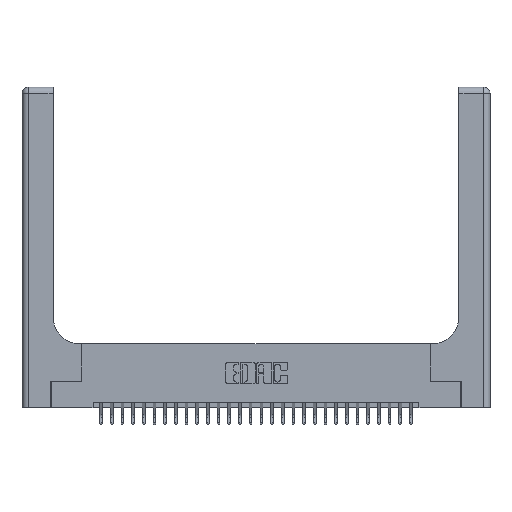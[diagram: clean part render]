
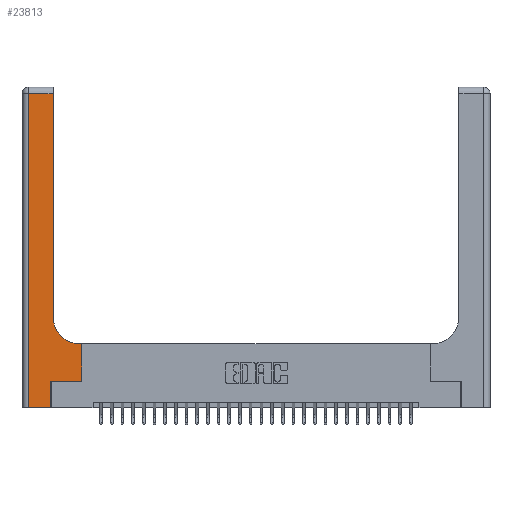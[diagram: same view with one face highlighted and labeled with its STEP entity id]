
A CAD part, top view. The second image highlights one B-rep face of the part: STEP entity #23813.
In plain terms, the highlighted planar face has unit normal (0, 0, 1).
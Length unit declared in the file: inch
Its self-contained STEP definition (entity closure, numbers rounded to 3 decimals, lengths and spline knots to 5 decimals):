
#58 = VERTEX_POINT ( 'NONE', #15473 ) ;
#102 = DIRECTION ( 'NONE',  ( 0., 1., 0. ) ) ;
#918 = AXIS2_PLACEMENT_3D ( 'NONE', #6945, #30186, #16162 ) ;
#1319 = CARTESIAN_POINT ( 'NONE',  ( 0.5415, 0.6, 0.37 ) ) ;
#1729 = CARTESIAN_POINT ( 'NONE',  ( 0.06, 3., 0.37 ) ) ;
#1959 = LINE ( 'NONE', #2387, #11537 ) ;
#2387 = CARTESIAN_POINT ( 'NONE',  ( 0.5585, 0.25, 0.37 ) ) ;
#2686 = VERTEX_POINT ( 'NONE', #16054 ) ;
#3421 = EDGE_LOOP ( 'NONE', ( #17281, #29422, #12052, #12313, #5362, #10881, #8377, #27648, #24285 ) ) ;
#3816 = CARTESIAN_POINT ( 'NONE',  ( 0.269, 0., 0.37 ) ) ;
#3995 = CIRCLE ( 'NONE', #918, 0.25 ) ;
#4967 = EDGE_CURVE ( 'NONE', #2686, #8994, #1959, .T. ) ;
#5325 = CARTESIAN_POINT ( 'NONE',  ( 0., 3., 0.37 ) ) ;
#5335 = EDGE_CURVE ( 'NONE', #58, #2686, #25581, .T. ) ;
#5362 = ORIENTED_EDGE ( 'NONE', *, *, #17693, .T. ) ;
#5519 = VECTOR ( 'NONE', #22151, 39.37008 ) ;
#5644 = CARTESIAN_POINT ( 'NONE',  ( 0., 0., 0.37 ) ) ;
#6528 = DIRECTION ( 'NONE',  ( -1., 0., 0. ) ) ;
#6945 = CARTESIAN_POINT ( 'NONE',  ( 0.5415, 0.85, 0.37 ) ) ;
#7024 = AXIS2_PLACEMENT_3D ( 'NONE', #5325, #24428, #22042 ) ;
#7540 = EDGE_CURVE ( 'NONE', #8994, #11600, #23949, .T. ) ;
#7541 = DIRECTION ( 'NONE',  ( 0., 1., 0. ) ) ;
#7999 = FACE_OUTER_BOUND ( 'NONE', #3421, .T. ) ;
#8024 = CARTESIAN_POINT ( 'NONE',  ( 0.269, 0.25, 0.37 ) ) ;
#8218 = VERTEX_POINT ( 'NONE', #3816 ) ;
#8377 = ORIENTED_EDGE ( 'NONE', *, *, #4967, .T. ) ;
#8994 = VERTEX_POINT ( 'NONE', #23214 ) ;
#9648 = VERTEX_POINT ( 'NONE', #19683 ) ;
#10881 = ORIENTED_EDGE ( 'NONE', *, *, #5335, .T. ) ;
#11537 = VECTOR ( 'NONE', #14271, 39.37008 ) ;
#11600 = VERTEX_POINT ( 'NONE', #1319 ) ;
#11716 = DIRECTION ( 'NONE',  ( -1., 0., 0. ) ) ;
#11780 = LINE ( 'NONE', #16689, #28784 ) ;
#12052 = ORIENTED_EDGE ( 'NONE', *, *, #28576, .T. ) ;
#12303 = CARTESIAN_POINT ( 'NONE',  ( 0.269, 0., 0.37 ) ) ;
#12313 = ORIENTED_EDGE ( 'NONE', *, *, #30443, .T. ) ;
#13387 = CARTESIAN_POINT ( 'NONE',  ( 0.2915, 0.6, 0.37 ) ) ;
#13583 = CARTESIAN_POINT ( 'NONE',  ( 0.2915, 0.85, 0.37 ) ) ;
#13860 = LINE ( 'NONE', #25816, #16829 ) ;
#14271 = DIRECTION ( 'NONE',  ( 0., 1., 0. ) ) ;
#14491 = VECTOR ( 'NONE', #25168, 39.37008 ) ;
#15473 = CARTESIAN_POINT ( 'NONE',  ( 0.269, 0.25, 0.37 ) ) ;
#16054 = CARTESIAN_POINT ( 'NONE',  ( 0.5585, 0.25, 0.37 ) ) ;
#16162 = DIRECTION ( 'NONE',  ( 1., 0., 0. ) ) ;
#16615 = LINE ( 'NONE', #5644, #5519 ) ;
#16689 = CARTESIAN_POINT ( 'NONE',  ( 0., 2.94, 0.37 ) ) ;
#16749 = CARTESIAN_POINT ( 'NONE',  ( 0.06, 0., 0.37 ) ) ;
#16829 = VECTOR ( 'NONE', #102, 39.37008 ) ;
#16939 = VECTOR ( 'NONE', #6528, 39.37008 ) ;
#17230 = VERTEX_POINT ( 'NONE', #13583 ) ;
#17281 = ORIENTED_EDGE ( 'NONE', *, *, #24957, .T. ) ;
#17693 = EDGE_CURVE ( 'NONE', #8218, #58, #19782, .T. ) ;
#19366 = PLANE ( 'NONE',  #7024 ) ;
#19683 = CARTESIAN_POINT ( 'NONE',  ( 0.06, 2.94, 0.37 ) ) ;
#19782 = LINE ( 'NONE', #12303, #24573 ) ;
#20290 = VECTOR ( 'NONE', #20823, 39.37008 ) ;
#20823 = DIRECTION ( 'NONE',  ( 0., -1., 0. ) ) ;
#22042 = DIRECTION ( 'NONE',  ( -1., 0., 0. ) ) ;
#22151 = DIRECTION ( 'NONE',  ( 1., 0., 0. ) ) ;
#23214 = CARTESIAN_POINT ( 'NONE',  ( 0.5585, 0.6, 0.37 ) ) ;
#23813 = ADVANCED_FACE ( 'NONE', ( #7999 ), #19366, .F. ) ;
#23949 = LINE ( 'NONE', #13387, #16939 ) ;
#24285 = ORIENTED_EDGE ( 'NONE', *, *, #29411, .T. ) ;
#24428 = DIRECTION ( 'NONE',  ( 0., 0., -1. ) ) ;
#24573 = VECTOR ( 'NONE', #7541, 39.37008 ) ;
#24957 = EDGE_CURVE ( 'NONE', #17230, #25185, #13860, .T. ) ;
#25168 = DIRECTION ( 'NONE',  ( 1., 0., 0. ) ) ;
#25185 = VERTEX_POINT ( 'NONE', #29933 ) ;
#25581 = LINE ( 'NONE', #8024, #14491 ) ;
#25816 = CARTESIAN_POINT ( 'NONE',  ( 0.2915, 3., 0.37 ) ) ;
#27288 = LINE ( 'NONE', #1729, #20290 ) ;
#27575 = VERTEX_POINT ( 'NONE', #16749 ) ;
#27648 = ORIENTED_EDGE ( 'NONE', *, *, #7540, .T. ) ;
#28576 = EDGE_CURVE ( 'NONE', #9648, #27575, #27288, .T. ) ;
#28732 = EDGE_CURVE ( 'NONE', #25185, #9648, #11780, .T. ) ;
#28784 = VECTOR ( 'NONE', #11716, 39.37008 ) ;
#29411 = EDGE_CURVE ( 'NONE', #11600, #17230, #3995, .T. ) ;
#29422 = ORIENTED_EDGE ( 'NONE', *, *, #28732, .T. ) ;
#29933 = CARTESIAN_POINT ( 'NONE',  ( 0.2915, 2.94, 0.37 ) ) ;
#30186 = DIRECTION ( 'NONE',  ( 0., 0., -1. ) ) ;
#30443 = EDGE_CURVE ( 'NONE', #27575, #8218, #16615, .T. ) ;
